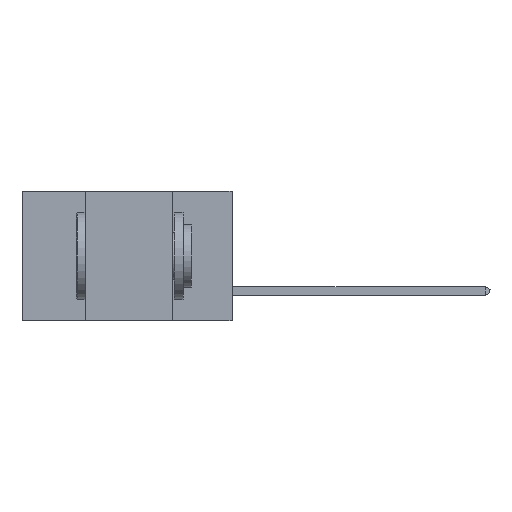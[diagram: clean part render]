
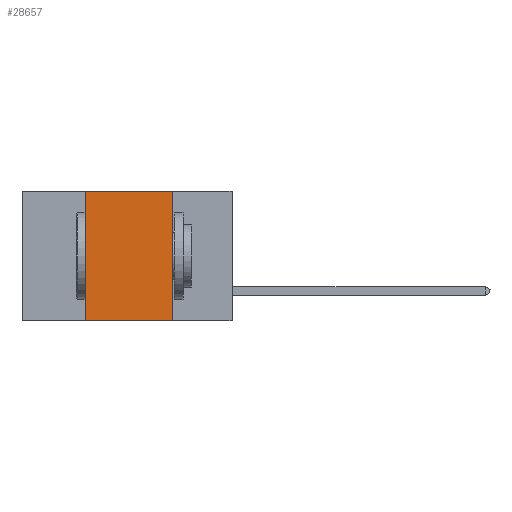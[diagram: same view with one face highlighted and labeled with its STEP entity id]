
A CAD part, left-side view. The second image highlights one B-rep face of the part: STEP entity #28657.
In plain terms, the highlighted planar face has unit normal (-1, 0, 0).
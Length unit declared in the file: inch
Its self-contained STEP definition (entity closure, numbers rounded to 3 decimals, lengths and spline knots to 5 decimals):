
#1310 = LINE ( 'NONE', #12976, #2042 ) ;
#2042 = VECTOR ( 'NONE', #20329, 39.37008 ) ;
#2464 = LINE ( 'NONE', #19023, #27152 ) ;
#3007 = VERTEX_POINT ( 'NONE', #29605 ) ;
#3047 = AXIS2_PLACEMENT_3D ( 'NONE', #8953, #11461, #13544 ) ;
#8445 = ORIENTED_EDGE ( 'NONE', *, *, #24601, .F. ) ;
#8953 = CARTESIAN_POINT ( 'NONE',  ( 0., 0.6, 0. ) ) ;
#9161 = PLANE ( 'NONE',  #3047 ) ;
#9561 = VERTEX_POINT ( 'NONE', #11154 ) ;
#10219 = EDGE_CURVE ( 'NONE', #15834, #9561, #19592, .T. ) ;
#10785 = VERTEX_POINT ( 'NONE', #19428 ) ;
#11154 = CARTESIAN_POINT ( 'NONE',  ( 0., 0.17, 0. ) ) ;
#11461 = DIRECTION ( 'NONE',  ( 1., 0., 0. ) ) ;
#11866 = CARTESIAN_POINT ( 'NONE',  ( 0., 0.42, 0. ) ) ;
#12969 = DIRECTION ( 'NONE',  ( 0., 0., -1. ) ) ;
#12976 = CARTESIAN_POINT ( 'NONE',  ( 0., 0.42, 0. ) ) ;
#13544 = DIRECTION ( 'NONE',  ( 0., 0., -1. ) ) ;
#13667 = LINE ( 'NONE', #22310, #30089 ) ;
#13708 = VECTOR ( 'NONE', #15753, 39.37008 ) ;
#14493 = FACE_OUTER_BOUND ( 'NONE', #27397, .T. ) ;
#15753 = DIRECTION ( 'NONE',  ( 0., -1., 0. ) ) ;
#15834 = VERTEX_POINT ( 'NONE', #11866 ) ;
#16125 = ORIENTED_EDGE ( 'NONE', *, *, #10219, .F. ) ;
#16347 = DIRECTION ( 'NONE',  ( 0., -1., 0. ) ) ;
#19023 = CARTESIAN_POINT ( 'NONE',  ( 0., 0.6, -0.37 ) ) ;
#19428 = CARTESIAN_POINT ( 'NONE',  ( 0., 0.42, -0.37 ) ) ;
#19592 = LINE ( 'NONE', #24819, #13708 ) ;
#20329 = DIRECTION ( 'NONE',  ( 0., 0., 1. ) ) ;
#20664 = ORIENTED_EDGE ( 'NONE', *, *, #22668, .F. ) ;
#21808 = EDGE_CURVE ( 'NONE', #10785, #3007, #2464, .T. ) ;
#22310 = CARTESIAN_POINT ( 'NONE',  ( 0., 0.17, 0. ) ) ;
#22668 = EDGE_CURVE ( 'NONE', #9561, #3007, #13667, .T. ) ;
#24601 = EDGE_CURVE ( 'NONE', #10785, #15834, #1310, .T. ) ;
#24819 = CARTESIAN_POINT ( 'NONE',  ( 0., 0.6, 0. ) ) ;
#26262 = ORIENTED_EDGE ( 'NONE', *, *, #21808, .T. ) ;
#27152 = VECTOR ( 'NONE', #16347, 39.37008 ) ;
#27397 = EDGE_LOOP ( 'NONE', ( #20664, #16125, #8445, #26262 ) ) ;
#28657 = ADVANCED_FACE ( 'NONE', ( #14493 ), #9161, .F. ) ;
#29605 = CARTESIAN_POINT ( 'NONE',  ( 0., 0.17, -0.37 ) ) ;
#30089 = VECTOR ( 'NONE', #12969, 39.37008 ) ;
